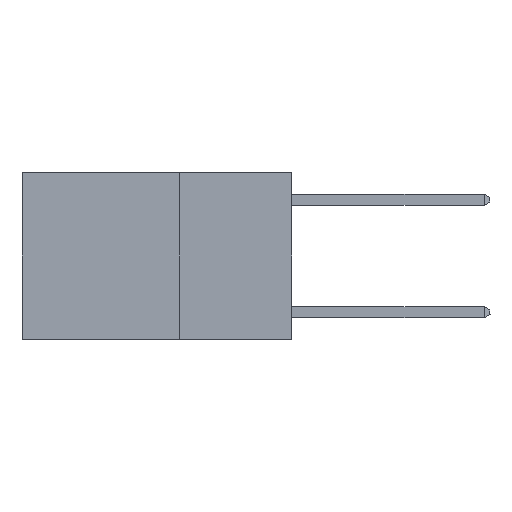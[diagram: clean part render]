
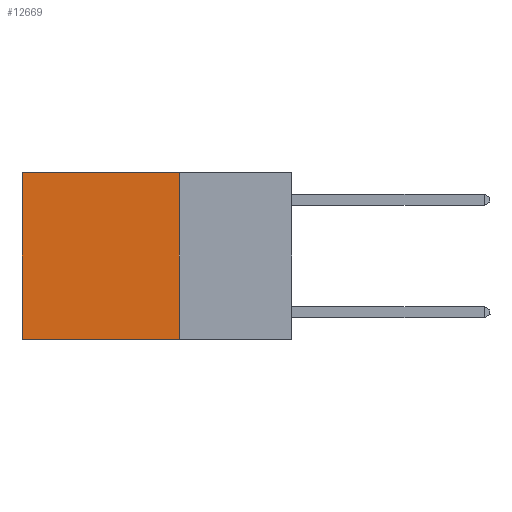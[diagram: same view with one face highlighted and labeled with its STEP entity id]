
A CAD part, left-side view. The second image highlights one B-rep face of the part: STEP entity #12669.
In plain terms, the highlighted planar face has unit normal (-1, 0, 0).
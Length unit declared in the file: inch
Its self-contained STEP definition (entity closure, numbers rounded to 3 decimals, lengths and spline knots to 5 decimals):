
#429 = LINE ( 'NONE', #4858, #3589 ) ;
#606 = EDGE_CURVE ( 'NONE', #12353, #2939, #3653, .T. ) ;
#1660 = EDGE_CURVE ( 'NONE', #2939, #12922, #7044, .T. ) ;
#1853 = FACE_OUTER_BOUND ( 'NONE', #10817, .T. ) ;
#2308 = DIRECTION ( 'NONE',  ( 0., 1., 0. ) ) ;
#2399 = VECTOR ( 'NONE', #13805, 39.37008 ) ;
#2686 = ORIENTED_EDGE ( 'NONE', *, *, #606, .F. ) ;
#2939 = VERTEX_POINT ( 'NONE', #7064 ) ;
#3495 = ORIENTED_EDGE ( 'NONE', *, *, #1660, .F. ) ;
#3551 = CARTESIAN_POINT ( 'NONE',  ( 0.2625, 0.25, -0.37 ) ) ;
#3589 = VECTOR ( 'NONE', #10618, 39.37008 ) ;
#3653 = LINE ( 'NONE', #10446, #6463 ) ;
#3734 = CARTESIAN_POINT ( 'NONE',  ( 0.2625, 0.6, -0.37 ) ) ;
#4479 = VERTEX_POINT ( 'NONE', #8680 ) ;
#4695 = LINE ( 'NONE', #11528, #2399 ) ;
#4819 = DIRECTION ( 'NONE',  ( 0., 0., -1. ) ) ;
#4858 = CARTESIAN_POINT ( 'NONE',  ( 0.2625, 0.6, 0. ) ) ;
#5057 = PLANE ( 'NONE',  #7134 ) ;
#5313 = ORIENTED_EDGE ( 'NONE', *, *, #8414, .T. ) ;
#5376 = ORIENTED_EDGE ( 'NONE', *, *, #9205, .T. ) ;
#6284 = CARTESIAN_POINT ( 'NONE',  ( 0.2625, 0.25, 0. ) ) ;
#6463 = VECTOR ( 'NONE', #4819, 39.37008 ) ;
#7044 = LINE ( 'NONE', #3551, #11589 ) ;
#7064 = CARTESIAN_POINT ( 'NONE',  ( 0.2625, 0.25, -0.37 ) ) ;
#7134 = AXIS2_PLACEMENT_3D ( 'NONE', #6284, #9728, #9431 ) ;
#8414 = EDGE_CURVE ( 'NONE', #12353, #4479, #4695, .T. ) ;
#8680 = CARTESIAN_POINT ( 'NONE',  ( 0.2625, 0.6, 0. ) ) ;
#9205 = EDGE_CURVE ( 'NONE', #4479, #12922, #429, .T. ) ;
#9431 = DIRECTION ( 'NONE',  ( 0., 0., -1. ) ) ;
#9728 = DIRECTION ( 'NONE',  ( 1., 0., 0. ) ) ;
#9886 = CARTESIAN_POINT ( 'NONE',  ( 0.2625, 0.25, 0. ) ) ;
#10446 = CARTESIAN_POINT ( 'NONE',  ( 0.2625, 0.25, 0. ) ) ;
#10618 = DIRECTION ( 'NONE',  ( 0., 0., -1. ) ) ;
#10817 = EDGE_LOOP ( 'NONE', ( #5376, #3495, #2686, #5313 ) ) ;
#11528 = CARTESIAN_POINT ( 'NONE',  ( 0.2625, 0.25, 0. ) ) ;
#11589 = VECTOR ( 'NONE', #2308, 39.37008 ) ;
#12353 = VERTEX_POINT ( 'NONE', #9886 ) ;
#12669 = ADVANCED_FACE ( 'NONE', ( #1853 ), #5057, .F. ) ;
#12922 = VERTEX_POINT ( 'NONE', #3734 ) ;
#13805 = DIRECTION ( 'NONE',  ( 0., 1., 0. ) ) ;
